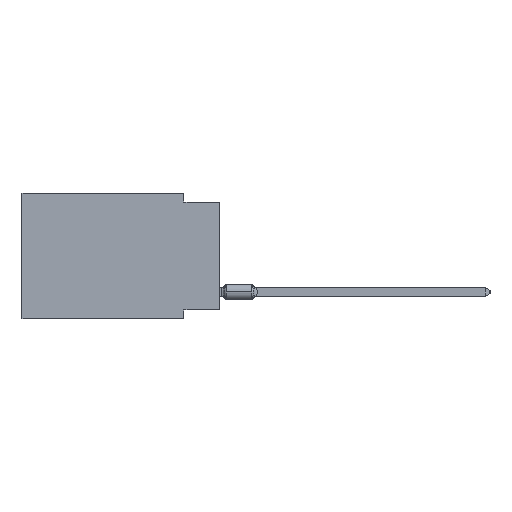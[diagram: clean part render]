
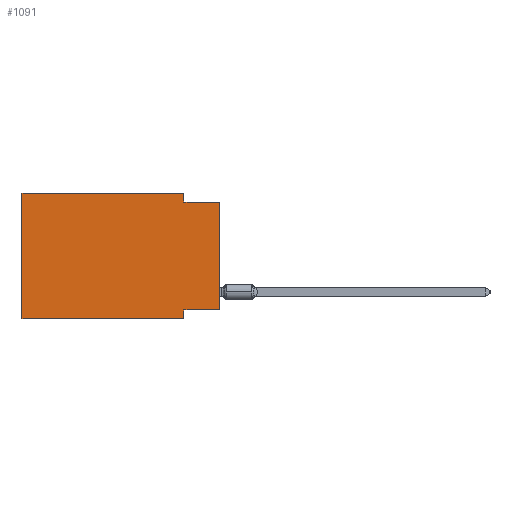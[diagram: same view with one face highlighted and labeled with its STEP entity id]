
A CAD part, left-side view. The second image highlights one B-rep face of the part: STEP entity #1091.
In plain terms, the highlighted planar face has unit normal (-1, 0, 0).
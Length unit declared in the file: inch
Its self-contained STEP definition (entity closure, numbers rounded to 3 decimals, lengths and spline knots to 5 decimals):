
#700 = DIRECTION ( 'NONE',  ( 0., 0., -1. ) ) ;
#1091 = ADVANCED_FACE ( 'NONE', ( #35598 ), #1260, .F. ) ;
#1260 = PLANE ( 'NONE',  #10115 ) ;
#1829 = CARTESIAN_POINT ( 'NONE',  ( 0., 0.55, 0. ) ) ;
#2487 = ORIENTED_EDGE ( 'NONE', *, *, #105010, .T. ) ;
#2574 = VERTEX_POINT ( 'NONE', #36552 ) ;
#4470 = EDGE_CURVE ( 'NONE', #2574, #52081, #103774, .T. ) ;
#5514 = CARTESIAN_POINT ( 'NONE',  ( 0., 0.55, 0. ) ) ;
#7841 = DIRECTION ( 'NONE',  ( 0., 0., -1. ) ) ;
#8497 = DIRECTION ( 'NONE',  ( 0., 0., -1. ) ) ;
#10115 = AXIS2_PLACEMENT_3D ( 'NONE', #1829, #96331, #700 ) ;
#11298 = EDGE_LOOP ( 'NONE', ( #2487, #101692, #65304, #20375, #62738, #43198, #87014, #66584 ) ) ;
#14836 = CARTESIAN_POINT ( 'NONE',  ( 0., 0.1, 0. ) ) ;
#17054 = VECTOR ( 'NONE', #26880, 39.37008 ) ;
#20375 = ORIENTED_EDGE ( 'NONE', *, *, #51466, .F. ) ;
#20829 = CARTESIAN_POINT ( 'NONE',  ( 0., 0.55, -0.35 ) ) ;
#21723 = CARTESIAN_POINT ( 'NONE',  ( 0., 0., -0.025 ) ) ;
#21891 = VECTOR ( 'NONE', #90711, 39.37008 ) ;
#22160 = CARTESIAN_POINT ( 'NONE',  ( 0., 0.55, 0. ) ) ;
#22364 = VECTOR ( 'NONE', #8497, 39.37008 ) ;
#24456 = LINE ( 'NONE', #86872, #113129 ) ;
#25027 = CARTESIAN_POINT ( 'NONE',  ( 0., 0.1, -0.025 ) ) ;
#26880 = DIRECTION ( 'NONE',  ( 0., 0., 1. ) ) ;
#30755 = LINE ( 'NONE', #22160, #60011 ) ;
#31104 = LINE ( 'NONE', #20829, #21891 ) ;
#31918 = VERTEX_POINT ( 'NONE', #50317 ) ;
#33109 = LINE ( 'NONE', #57820, #96182 ) ;
#35598 = FACE_OUTER_BOUND ( 'NONE', #11298, .T. ) ;
#36552 = CARTESIAN_POINT ( 'NONE',  ( 0., 0., -0.325 ) ) ;
#40400 = VERTEX_POINT ( 'NONE', #112795 ) ;
#40480 = DIRECTION ( 'NONE',  ( 0., 0., 1. ) ) ;
#41525 = EDGE_CURVE ( 'NONE', #60703, #95685, #31104, .T. ) ;
#43198 = ORIENTED_EDGE ( 'NONE', *, *, #41525, .T. ) ;
#44644 = LINE ( 'NONE', #104244, #17054 ) ;
#47333 = DIRECTION ( 'NONE',  ( 0., -1., 0. ) ) ;
#47755 = EDGE_CURVE ( 'NONE', #52081, #95685, #24456, .T. ) ;
#49884 = VERTEX_POINT ( 'NONE', #25027 ) ;
#50317 = CARTESIAN_POINT ( 'NONE',  ( 0., 0.55, 0. ) ) ;
#51466 = EDGE_CURVE ( 'NONE', #31918, #40400, #83982, .T. ) ;
#52081 = VERTEX_POINT ( 'NONE', #112969 ) ;
#57820 = CARTESIAN_POINT ( 'NONE',  ( 0., 0., -0.025 ) ) ;
#59523 = LINE ( 'NONE', #14836, #22364 ) ;
#60011 = VECTOR ( 'NONE', #40480, 39.37008 ) ;
#60703 = VERTEX_POINT ( 'NONE', #98585 ) ;
#61381 = CARTESIAN_POINT ( 'NONE',  ( 0., 0., -0.325 ) ) ;
#62738 = ORIENTED_EDGE ( 'NONE', *, *, #87894, .F. ) ;
#64247 = VERTEX_POINT ( 'NONE', #21723 ) ;
#64374 = EDGE_CURVE ( 'NONE', #49884, #64247, #33109, .T. ) ;
#65304 = ORIENTED_EDGE ( 'NONE', *, *, #77438, .F. ) ;
#66584 = ORIENTED_EDGE ( 'NONE', *, *, #4470, .F. ) ;
#71229 = VECTOR ( 'NONE', #77450, 39.37008 ) ;
#77438 = EDGE_CURVE ( 'NONE', #40400, #49884, #59523, .T. ) ;
#77450 = DIRECTION ( 'NONE',  ( 0., 1., 0. ) ) ;
#79497 = CARTESIAN_POINT ( 'NONE',  ( 0., 0.1, -0.35 ) ) ;
#83982 = LINE ( 'NONE', #5514, #106163 ) ;
#86872 = CARTESIAN_POINT ( 'NONE',  ( 0., 0.1, -0.35 ) ) ;
#87014 = ORIENTED_EDGE ( 'NONE', *, *, #47755, .F. ) ;
#87894 = EDGE_CURVE ( 'NONE', #60703, #31918, #30755, .T. ) ;
#90711 = DIRECTION ( 'NONE',  ( 0., -1., 0. ) ) ;
#92177 = DIRECTION ( 'NONE',  ( 0., -1., 0. ) ) ;
#95685 = VERTEX_POINT ( 'NONE', #79497 ) ;
#96182 = VECTOR ( 'NONE', #92177, 39.37008 ) ;
#96331 = DIRECTION ( 'NONE',  ( 1., 0., 0. ) ) ;
#98585 = CARTESIAN_POINT ( 'NONE',  ( 0., 0.55, -0.35 ) ) ;
#101692 = ORIENTED_EDGE ( 'NONE', *, *, #64374, .F. ) ;
#103774 = LINE ( 'NONE', #61381, #71229 ) ;
#104244 = CARTESIAN_POINT ( 'NONE',  ( 0., 0., 0. ) ) ;
#105010 = EDGE_CURVE ( 'NONE', #2574, #64247, #44644, .T. ) ;
#106163 = VECTOR ( 'NONE', #47333, 39.37008 ) ;
#112795 = CARTESIAN_POINT ( 'NONE',  ( 0., 0.1, 0. ) ) ;
#112969 = CARTESIAN_POINT ( 'NONE',  ( 0., 0.1, -0.325 ) ) ;
#113129 = VECTOR ( 'NONE', #7841, 39.37008 ) ;
